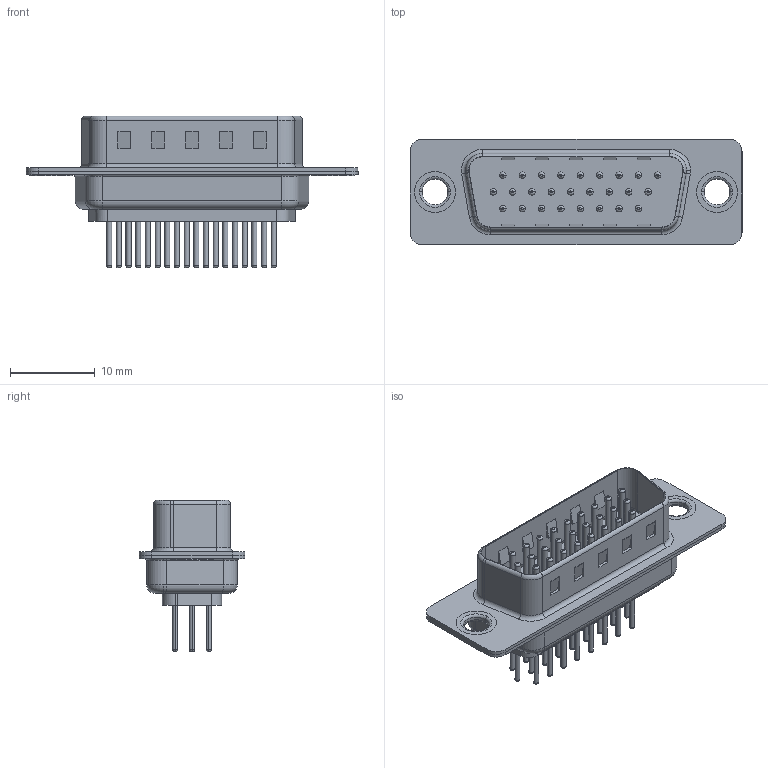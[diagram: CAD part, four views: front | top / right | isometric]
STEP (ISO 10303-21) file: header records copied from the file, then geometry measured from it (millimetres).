
FILE_DESCRIPTION (( 'STEP AP203' ), '1' );
FILE_NAME ('637-M26-630-BT1.STEP', '2018-11-20T00:08:17', ( '' ), ( '' ), 'SwSTEP 2.0', 'SolidWorks 2016', '' );
FILE_SCHEMA (( 'CONFIG_CONTROL_DESIGN' ));
Length unit declared in the file: millimetre
Products named in the file (8): 637M Contact Row 1_30; 637M Contact Row 2_30; 637M Contact Row 3_30; 637M Thru Hole Rivet; 637-M26-630-BT1; 637M Housing_26 Contacts; 637M Shell Front_26 Contacts; 637M Shell Rear_26 Contacts
Assembly tree (31 placements, depth 2):
  637-M26-630-BT1
    637M Housing_26 Contacts
    637M Shell Front_26 Contacts
    637M Shell Rear_26 Contacts
    637M Contact Row 1_30  x9
    637M Contact Row 2_30  x9
    637M Contact Row 3_30  x8
    637M Thru Hole Rivet  x2
Bounding box: 39.2 x 12.5 x 17.9 mm (x, y, z)
Volume: 1831 mm3; surface area: 5605.5 mm2
Topology: 31 solids, 31 shells, 1276 faces, 2699 edges, 1626 vertices
Faces by surface type: cylinder 481, torus 474, plane 321
Entity records: 18779 total; most frequent: DIRECTION 3343, CARTESIAN_POINT 2925, ORIENTED_EDGE 2742, EDGE_CURVE 1371, AXIS2_PLACEMENT_3D 1364, VERTEX_POINT 866, EDGE_LOOP 745, CIRCLE 741
